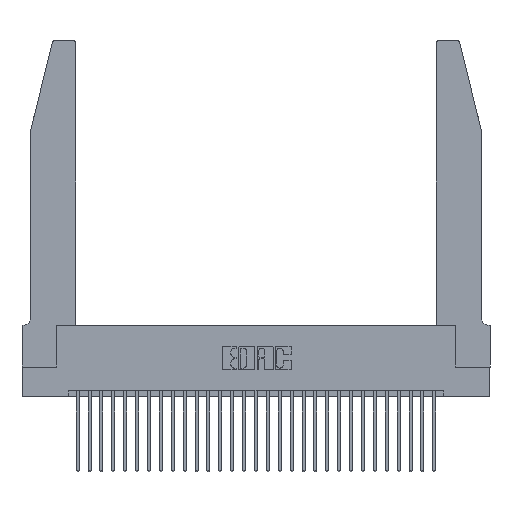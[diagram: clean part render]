
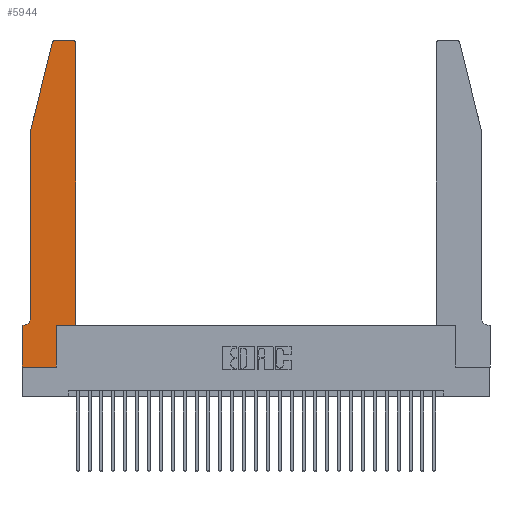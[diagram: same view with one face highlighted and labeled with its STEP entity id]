
A CAD part, top view. The second image highlights one B-rep face of the part: STEP entity #5944.
In plain terms, the highlighted planar face has unit normal (0, 0, 1).
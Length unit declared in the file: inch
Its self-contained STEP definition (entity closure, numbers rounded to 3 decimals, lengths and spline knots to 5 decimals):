
#273 = DIRECTION ( 'NONE',  ( 0., 0., 1. ) ) ;
#366 = AXIS2_PLACEMENT_3D ( 'NONE', #14415, #273, #16982 ) ;
#1438 = VERTEX_POINT ( 'NONE', #17019 ) ;
#2131 = DIRECTION ( 'NONE',  ( 1., 0., 0. ) ) ;
#2175 = CIRCLE ( 'NONE', #4273, 0.07 ) ;
#2941 = ORIENTED_EDGE ( 'NONE', *, *, #25055, .T. ) ;
#2996 = CARTESIAN_POINT ( 'NONE',  ( 0.0755, 2., 0.37 ) ) ;
#4202 = VECTOR ( 'NONE', #21015, 39.37008 ) ;
#4273 = AXIS2_PLACEMENT_3D ( 'NONE', #23763, #9662, #26116 ) ;
#5257 = CARTESIAN_POINT ( 'NONE',  ( 0.4205, 2.75, 0.37 ) ) ;
#5644 = CARTESIAN_POINT ( 'NONE',  ( 0.0755, 0.42, 0.37 ) ) ;
#5943 = VERTEX_POINT ( 'NONE', #26289 ) ;
#5944 = ADVANCED_FACE ( 'NONE', ( #26658 ), #14616, .T. ) ;
#5947 = VERTEX_POINT ( 'NONE', #12210 ) ;
#6673 = ORIENTED_EDGE ( 'NONE', *, *, #25921, .T. ) ;
#6841 = CARTESIAN_POINT ( 'NONE',  ( 0.4205, 2.72, 0.37 ) ) ;
#7397 = VERTEX_POINT ( 'NONE', #22242 ) ;
#7924 = VECTOR ( 'NONE', #25933, 39.37008 ) ;
#8366 = EDGE_CURVE ( 'NONE', #26019, #23264, #2175, .T. ) ;
#8423 = DIRECTION ( 'NONE',  ( 0., 0., 1. ) ) ;
#8468 = VECTOR ( 'NONE', #28886, 39.37008 ) ;
#8921 = VERTEX_POINT ( 'NONE', #16466 ) ;
#9050 = VECTOR ( 'NONE', #2131, 39.37008 ) ;
#9086 = VECTOR ( 'NONE', #13411, 39.37008 ) ;
#9154 = EDGE_CURVE ( 'NONE', #5947, #8921, #14804, .T. ) ;
#9243 = DIRECTION ( 'NONE',  ( 1., 0., 0. ) ) ;
#9662 = DIRECTION ( 'NONE',  ( 0., 0., -1. ) ) ;
#10318 = VECTOR ( 'NONE', #24475, 39.37008 ) ;
#10332 = ORIENTED_EDGE ( 'NONE', *, *, #15373, .T. ) ;
#10388 = CARTESIAN_POINT ( 'NONE',  ( 0.0755, 2., 0.37 ) ) ;
#11048 = LINE ( 'NONE', #10388, #10318 ) ;
#11566 = DIRECTION ( 'NONE',  ( -1., 0., 0. ) ) ;
#11799 = LINE ( 'NONE', #23304, #17349 ) ;
#12210 = CARTESIAN_POINT ( 'NONE',  ( 0.2865, 0., 0.37 ) ) ;
#12306 = VECTOR ( 'NONE', #12494, 39.37008 ) ;
#12447 = CIRCLE ( 'NONE', #18224, 0.03 ) ;
#12494 = DIRECTION ( 'NONE',  ( 0., -1., 0. ) ) ;
#13411 = DIRECTION ( 'NONE',  ( 0., -1., 0. ) ) ;
#14221 = VERTEX_POINT ( 'NONE', #5257 ) ;
#14415 = CARTESIAN_POINT ( 'NONE',  ( 0., 0.35, 0.37 ) ) ;
#14616 = PLANE ( 'NONE',  #366 ) ;
#14804 = LINE ( 'NONE', #19529, #8468 ) ;
#14852 = ORIENTED_EDGE ( 'NONE', *, *, #18996, .T. ) ;
#15024 = VECTOR ( 'NONE', #25945, 39.37008 ) ;
#15311 = VERTEX_POINT ( 'NONE', #23255 ) ;
#15335 = EDGE_CURVE ( 'NONE', #7397, #25250, #16852, .T. ) ;
#15373 = EDGE_CURVE ( 'NONE', #8921, #7397, #15379, .T. ) ;
#15379 = LINE ( 'NONE', #23360, #9050 ) ;
#16466 = CARTESIAN_POINT ( 'NONE',  ( 0.2865, 0.35, 0.37 ) ) ;
#16513 = LINE ( 'NONE', #23600, #15024 ) ;
#16852 = LINE ( 'NONE', #30268, #4202 ) ;
#16982 = DIRECTION ( 'NONE',  ( 1., 0., 0. ) ) ;
#17019 = CARTESIAN_POINT ( 'NONE',  ( 0.0755, 2., 0.37 ) ) ;
#17184 = CIRCLE ( 'NONE', #29964, 0.03 ) ;
#17349 = VECTOR ( 'NONE', #11566, 39.37008 ) ;
#18224 = AXIS2_PLACEMENT_3D ( 'NONE', #22539, #8423, #24905 ) ;
#18996 = EDGE_CURVE ( 'NONE', #23264, #5943, #11799, .T. ) ;
#19529 = CARTESIAN_POINT ( 'NONE',  ( 0.2865, 0.35, 0.37 ) ) ;
#19715 = ORIENTED_EDGE ( 'NONE', *, *, #22175, .T. ) ;
#21015 = DIRECTION ( 'NONE',  ( 0., 1., 0. ) ) ;
#21623 = ORIENTED_EDGE ( 'NONE', *, *, #8366, .T. ) ;
#22009 = ORIENTED_EDGE ( 'NONE', *, *, #23568, .T. ) ;
#22175 = EDGE_CURVE ( 'NONE', #29293, #1438, #11048, .T. ) ;
#22242 = CARTESIAN_POINT ( 'NONE',  ( 0.4505, 0.35, 0.37 ) ) ;
#22539 = CARTESIAN_POINT ( 'NONE',  ( 0.284, 2.72, 0.37 ) ) ;
#22768 = CARTESIAN_POINT ( 'NONE',  ( 0., 0., 0.37 ) ) ;
#23255 = CARTESIAN_POINT ( 'NONE',  ( 0., 0., 0.37 ) ) ;
#23264 = VERTEX_POINT ( 'NONE', #23865 ) ;
#23304 = CARTESIAN_POINT ( 'NONE',  ( 0.0755, 0.35, 0.37 ) ) ;
#23356 = DIRECTION ( 'NONE',  ( 0., 0., 1. ) ) ;
#23360 = CARTESIAN_POINT ( 'NONE',  ( 0.4505, 0.35, 0.37 ) ) ;
#23568 = EDGE_CURVE ( 'NONE', #25376, #29293, #12447, .T. ) ;
#23600 = CARTESIAN_POINT ( 'NONE',  ( 0., 0., 0.37 ) ) ;
#23631 = ORIENTED_EDGE ( 'NONE', *, *, #28837, .T. ) ;
#23763 = CARTESIAN_POINT ( 'NONE',  ( 0.0055, 0.42, 0.37 ) ) ;
#23865 = CARTESIAN_POINT ( 'NONE',  ( 0.0055, 0.35, 0.37 ) ) ;
#24164 = CARTESIAN_POINT ( 'NONE',  ( 0.4505, 2.72, 0.37 ) ) ;
#24475 = DIRECTION ( 'NONE',  ( -0.239, -0.971, 0. ) ) ;
#24713 = EDGE_CURVE ( 'NONE', #14221, #25376, #25999, .T. ) ;
#24905 = DIRECTION ( 'NONE',  ( 1., 0., 0. ) ) ;
#24918 = ORIENTED_EDGE ( 'NONE', *, *, #28619, .T. ) ;
#25055 = EDGE_CURVE ( 'NONE', #25250, #14221, #17184, .T. ) ;
#25250 = VERTEX_POINT ( 'NONE', #24164 ) ;
#25376 = VERTEX_POINT ( 'NONE', #29334 ) ;
#25788 = ORIENTED_EDGE ( 'NONE', *, *, #15335, .T. ) ;
#25829 = CARTESIAN_POINT ( 'NONE',  ( 0.2605, 2.75, 0.37 ) ) ;
#25921 = EDGE_CURVE ( 'NONE', #1438, #26019, #30265, .T. ) ;
#25933 = DIRECTION ( 'NONE',  ( -1., 0., 0. ) ) ;
#25945 = DIRECTION ( 'NONE',  ( 1., 0., 0. ) ) ;
#25999 = LINE ( 'NONE', #25829, #7924 ) ;
#26019 = VERTEX_POINT ( 'NONE', #5644 ) ;
#26116 = DIRECTION ( 'NONE',  ( -1., 0., 0. ) ) ;
#26289 = CARTESIAN_POINT ( 'NONE',  ( 0., 0.35, 0.37 ) ) ;
#26658 = FACE_OUTER_BOUND ( 'NONE', #28866, .T. ) ;
#27627 = CARTESIAN_POINT ( 'NONE',  ( 0.25487, 2.72718, 0.37 ) ) ;
#28233 = ORIENTED_EDGE ( 'NONE', *, *, #9154, .T. ) ;
#28513 = ORIENTED_EDGE ( 'NONE', *, *, #24713, .T. ) ;
#28563 = LINE ( 'NONE', #22768, #9086 ) ;
#28619 = EDGE_CURVE ( 'NONE', #5943, #15311, #28563, .T. ) ;
#28837 = EDGE_CURVE ( 'NONE', #15311, #5947, #16513, .T. ) ;
#28866 = EDGE_LOOP ( 'NONE', ( #28513, #22009, #19715, #6673, #21623, #14852, #24918, #23631, #28233, #10332, #25788, #2941 ) ) ;
#28886 = DIRECTION ( 'NONE',  ( 0., 1., 0. ) ) ;
#29293 = VERTEX_POINT ( 'NONE', #27627 ) ;
#29334 = CARTESIAN_POINT ( 'NONE',  ( 0.284, 2.75, 0.37 ) ) ;
#29964 = AXIS2_PLACEMENT_3D ( 'NONE', #6841, #23356, #9243 ) ;
#30265 = LINE ( 'NONE', #2996, #12306 ) ;
#30268 = CARTESIAN_POINT ( 'NONE',  ( 0.4505, 0.35, 0.37 ) ) ;
